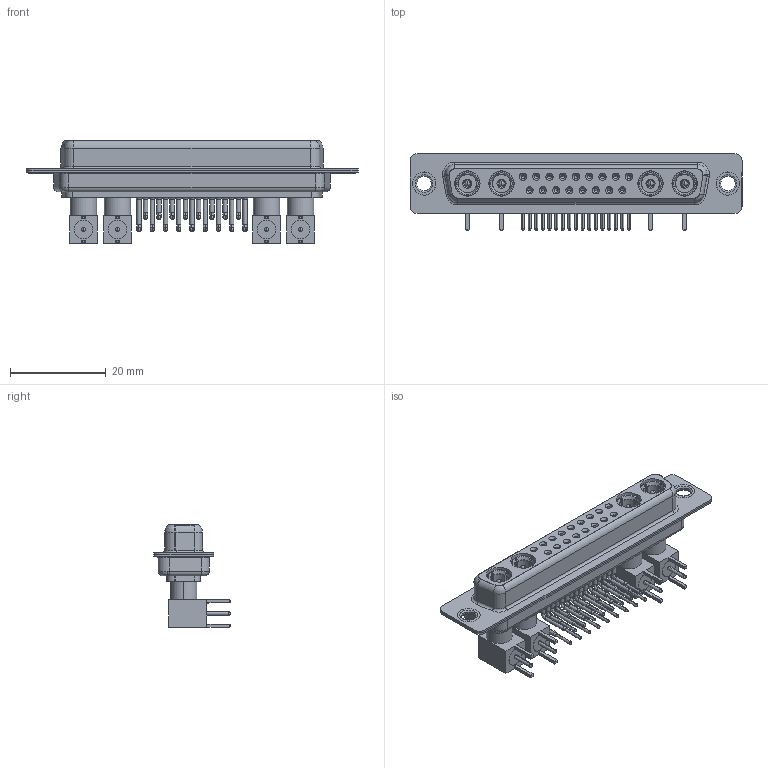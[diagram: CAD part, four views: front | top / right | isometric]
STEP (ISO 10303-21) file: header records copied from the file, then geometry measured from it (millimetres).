
FILE_DESCRIPTION (( 'STEP AP203' ), '1' );
FILE_NAME ('630-21W4640-5N1.STEP', '2022-06-08T18:40:59', ( '' ), ( '' ), 'SwSTEP 2.0', 'SolidWorks 2020', '' );
FILE_SCHEMA (( 'CONFIG_CONTROL_DESIGN' ));
Length unit declared in the file: millimetre
Products named in the file (17): Pin_RA; 630Combo Thru Hole Rivet; 630Combo Contact Row 1; RA Back Shell; 630Combo Housing_21W4; Insulator Pin_Straight PC Tail; Insulator RA Pin; 630Combo Shell Front_37 Contacts; Co-Ax Plug Assy_RA; 630Combo Contact Row 2; 630Combo Shell Rear_37 Contacts; Co-Ax Plug_RA PC Tail; Locking Collar; 630-21W4640-5N1
Assembly tree (50 placements, depth 3):
  630-21W4640-5N1
    630Combo Housing_21W4
    630Combo Shell Front_37 Contacts
    630Combo Shell Rear_37 Contacts
    630Combo Thru Hole Rivet  x2
    Co-Ax Plug Assy_RA
      Co-Ax Plug_RA PC Tail
      Insulator Pin_Straight PC Tail
      Pin_RA
      Locking Collar
      RA Back Shell
      Insulator RA Pin
    Co-Ax Plug Assy_RA
      Co-Ax Plug_RA PC Tail
      Insulator Pin_Straight PC Tail
      Pin_RA
      Locking Collar
      RA Back Shell
      Insulator RA Pin
    Co-Ax Plug Assy_RA
      Co-Ax Plug_RA PC Tail
      Insulator Pin_Straight PC Tail
      Pin_RA
      Locking Collar
      RA Back Shell
      Insulator RA Pin
    Co-Ax Plug Assy_RA
      Co-Ax Plug_RA PC Tail
      Insulator Pin_Straight PC Tail
      Pin_RA
      Locking Collar
      RA Back Shell
      Insulator RA Pin
    630Combo Contact Row 1  x9
    630Combo Contact Row 2  x8
Bounding box: 69.4 x 16 x 21.41 mm (x, y, z)
Volume: 6262.2 mm3; surface area: 14898.5 mm2
Topology: 46 solids, 46 shells, 1826 faces, 4502 edges, 2820 vertices
Faces by surface type: cylinder 772, plane 590, cone 287, torus 89, bspline 72, sphere 16
Entity records: 24110 total; most frequent: CARTESIAN_POINT 4101, DIRECTION 4009, ORIENTED_EDGE 3340, EDGE_CURVE 1670, AXIS2_PLACEMENT_3D 1661, VERTEX_POINT 1060, CIRCLE 896, EDGE_LOOP 864
